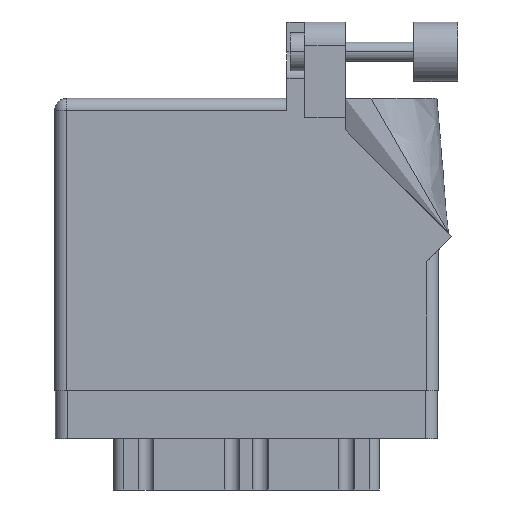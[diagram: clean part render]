
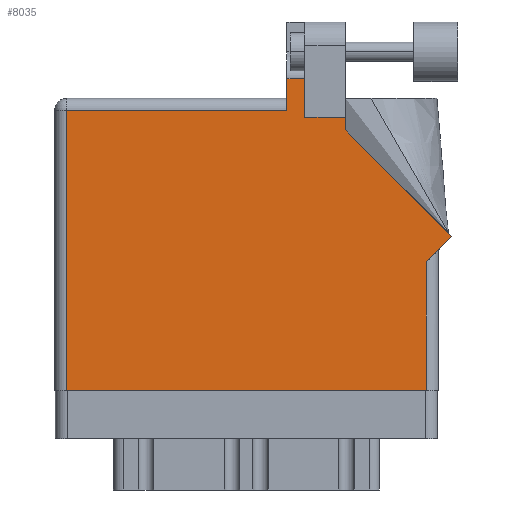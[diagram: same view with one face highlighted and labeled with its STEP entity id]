
A CAD part, front view. The second image highlights one B-rep face of the part: STEP entity #8035.
In plain terms, the highlighted face is planar.
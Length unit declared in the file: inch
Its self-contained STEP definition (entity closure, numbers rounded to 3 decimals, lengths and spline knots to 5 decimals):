
#97 = VECTOR ( 'NONE', #17432, 39.37008 ) ;
#521 = LINE ( 'NONE', #3346, #6241 ) ;
#552 = DIRECTION ( 'NONE',  ( -1., 0., 0. ) ) ;
#1364 = CARTESIAN_POINT ( 'NONE',  ( 1.311, 1.43, 0. ) ) ;
#1626 = CARTESIAN_POINT ( 'NONE',  ( 1.64177, 1.6315, 0. ) ) ;
#1706 = CARTESIAN_POINT ( 'NONE',  ( 1.948, 0.737, 0. ) ) ;
#2049 = VERTEX_POINT ( 'NONE', #31434 ) ;
#2344 = ORIENTED_EDGE ( 'NONE', *, *, #8327, .T. ) ;
#2584 = DIRECTION ( 'NONE',  ( 0., 1., 0. ) ) ;
#2872 = LINE ( 'NONE', #13479, #25493 ) ;
#3346 = CARTESIAN_POINT ( 'NONE',  ( 1.524, 1.43, 0. ) ) ;
#3378 = PLANE ( 'NONE',  #11171 ) ;
#3548 = EDGE_CURVE ( 'NONE', #6513, #9040, #521, .T. ) ;
#4272 = DIRECTION ( 'NONE',  ( -1., 0., 0. ) ) ;
#5540 = LINE ( 'NONE', #10955, #11343 ) ;
#6228 = VECTOR ( 'NONE', #10906, 39.37008 ) ;
#6241 = VECTOR ( 'NONE', #16433, 39.37008 ) ;
#6287 = EDGE_CURVE ( 'NONE', #28083, #24805, #22618, .T. ) ;
#6513 = VERTEX_POINT ( 'NONE', #28348 ) ;
#7803 = VECTOR ( 'NONE', #4272, 39.37008 ) ;
#7869 = VERTEX_POINT ( 'NONE', #15797 ) ;
#8035 = ADVANCED_FACE ( 'NONE', ( #22303 ), #3378, .F. ) ;
#8327 = EDGE_CURVE ( 'NONE', #27288, #22173, #5540, .T. ) ;
#8966 = ORIENTED_EDGE ( 'NONE', *, *, #6287, .T. ) ;
#9005 = CARTESIAN_POINT ( 'NONE',  ( 2.08071, 0.80771, 0. ) ) ;
#9040 = VERTEX_POINT ( 'NONE', #1364 ) ;
#9177 = ORIENTED_EDGE ( 'NONE', *, *, #15667, .T. ) ;
#10225 = VERTEX_POINT ( 'NONE', #33382 ) ;
#10813 = VECTOR ( 'NONE', #2584, 39.37008 ) ;
#10906 = DIRECTION ( 'NONE',  ( -0.707, 0.707, 0. ) ) ;
#10910 = ORIENTED_EDGE ( 'NONE', *, *, #28732, .T. ) ;
#10955 = CARTESIAN_POINT ( 'NONE',  ( 1.217, 1.53, 0. ) ) ;
#11171 = AXIS2_PLACEMENT_3D ( 'NONE', #24775, #19463, #552 ) ;
#11343 = VECTOR ( 'NONE', #29201, 39.37008 ) ;
#11828 = DIRECTION ( 'NONE',  ( 1., 0., 0. ) ) ;
#11869 = DIRECTION ( 'NONE',  ( 0.707, 0.707, 0. ) ) ;
#12842 = CARTESIAN_POINT ( 'NONE',  ( 0.062, 0., 0. ) ) ;
#13138 = DIRECTION ( 'NONE',  ( -1., 0., 0. ) ) ;
#13479 = CARTESIAN_POINT ( 'NONE',  ( 0., 1.468, 0. ) ) ;
#14165 = CARTESIAN_POINT ( 'NONE',  ( 1.948, 0., 0. ) ) ;
#14216 = VECTOR ( 'NONE', #17974, 39.37008 ) ;
#15020 = CARTESIAN_POINT ( 'NONE',  ( 0., 0., 0. ) ) ;
#15236 = ORIENTED_EDGE ( 'NONE', *, *, #18518, .T. ) ;
#15253 = EDGE_CURVE ( 'NONE', #34768, #28083, #20917, .T. ) ;
#15336 = CARTESIAN_POINT ( 'NONE',  ( 1.524, 1.36442, 0. ) ) ;
#15398 = ORIENTED_EDGE ( 'NONE', *, *, #29350, .T. ) ;
#15667 = EDGE_CURVE ( 'NONE', #24805, #10225, #31062, .T. ) ;
#15797 = CARTESIAN_POINT ( 'NONE',  ( 1.311, 1.6315, 0. ) ) ;
#16214 = CARTESIAN_POINT ( 'NONE',  ( 2.08071, 0.80771, 0. ) ) ;
#16289 = ORIENTED_EDGE ( 'NONE', *, *, #3548, .T. ) ;
#16433 = DIRECTION ( 'NONE',  ( -1., 0., 0. ) ) ;
#17039 = EDGE_CURVE ( 'NONE', #9040, #7869, #18829, .T. ) ;
#17267 = VECTOR ( 'NONE', #11828, 39.37008 ) ;
#17355 = LINE ( 'NONE', #1626, #7803 ) ;
#17432 = DIRECTION ( 'NONE',  ( 0., 1., 0. ) ) ;
#17974 = DIRECTION ( 'NONE',  ( 0., 1., 0. ) ) ;
#18518 = EDGE_CURVE ( 'NONE', #10225, #25397, #33276, .T. ) ;
#18829 = LINE ( 'NONE', #34147, #10813 ) ;
#19459 = CARTESIAN_POINT ( 'NONE',  ( 2.01, 0.737, 0. ) ) ;
#19463 = DIRECTION ( 'NONE',  ( 0., 0., -1. ) ) ;
#19788 = CARTESIAN_POINT ( 'NONE',  ( 0.062, 1.468, 0. ) ) ;
#20917 = LINE ( 'NONE', #23758, #25500 ) ;
#21047 = CARTESIAN_POINT ( 'NONE',  ( 1.217, 1.6315, 0. ) ) ;
#22031 = LINE ( 'NONE', #16214, #6228 ) ;
#22173 = VERTEX_POINT ( 'NONE', #33160 ) ;
#22303 = FACE_OUTER_BOUND ( 'NONE', #23037, .T. ) ;
#22618 = LINE ( 'NONE', #15020, #17267 ) ;
#23037 = EDGE_LOOP ( 'NONE', ( #30201, #32673, #2344, #10910, #23596, #8966, #9177, #15236, #33797, #15398, #16289 ) ) ;
#23596 = ORIENTED_EDGE ( 'NONE', *, *, #15253, .T. ) ;
#23758 = CARTESIAN_POINT ( 'NONE',  ( 0.062, 0., 0. ) ) ;
#24775 = CARTESIAN_POINT ( 'NONE',  ( 0., 1.53, 0. ) ) ;
#24805 = VERTEX_POINT ( 'NONE', #14165 ) ;
#25065 = EDGE_CURVE ( 'NONE', #7869, #27288, #17355, .T. ) ;
#25397 = VERTEX_POINT ( 'NONE', #9005 ) ;
#25493 = VECTOR ( 'NONE', #13138, 39.37008 ) ;
#25500 = VECTOR ( 'NONE', #34574, 39.37008 ) ;
#26166 = VECTOR ( 'NONE', #11869, 39.37008 ) ;
#27288 = VERTEX_POINT ( 'NONE', #21047 ) ;
#27773 = EDGE_CURVE ( 'NONE', #25397, #2049, #22031, .T. ) ;
#28083 = VERTEX_POINT ( 'NONE', #12842 ) ;
#28348 = CARTESIAN_POINT ( 'NONE',  ( 1.524, 1.43, 0. ) ) ;
#28732 = EDGE_CURVE ( 'NONE', #22173, #34768, #2872, .T. ) ;
#29201 = DIRECTION ( 'NONE',  ( 0., -1., 0. ) ) ;
#29350 = EDGE_CURVE ( 'NONE', #2049, #6513, #31942, .T. ) ;
#30201 = ORIENTED_EDGE ( 'NONE', *, *, #17039, .T. ) ;
#31062 = LINE ( 'NONE', #1706, #97 ) ;
#31434 = CARTESIAN_POINT ( 'NONE',  ( 1.524, 1.36442, 0. ) ) ;
#31942 = LINE ( 'NONE', #15336, #14216 ) ;
#32673 = ORIENTED_EDGE ( 'NONE', *, *, #25065, .T. ) ;
#33160 = CARTESIAN_POINT ( 'NONE',  ( 1.217, 1.468, 0. ) ) ;
#33276 = LINE ( 'NONE', #19459, #26166 ) ;
#33382 = CARTESIAN_POINT ( 'NONE',  ( 1.948, 0.675, 0. ) ) ;
#33797 = ORIENTED_EDGE ( 'NONE', *, *, #27773, .T. ) ;
#34147 = CARTESIAN_POINT ( 'NONE',  ( 1.311, 1.43, 0. ) ) ;
#34574 = DIRECTION ( 'NONE',  ( 0., -1., 0. ) ) ;
#34768 = VERTEX_POINT ( 'NONE', #19788 ) ;
